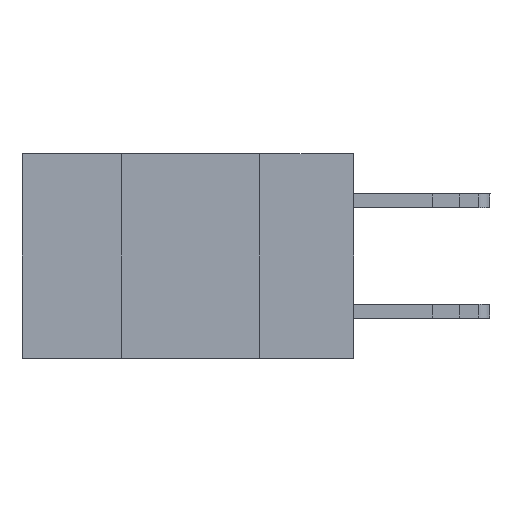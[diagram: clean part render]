
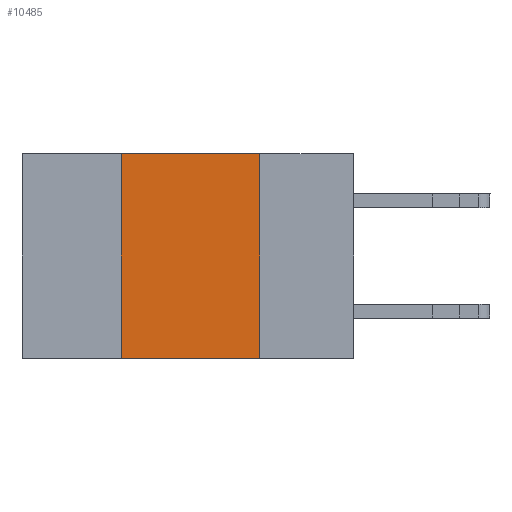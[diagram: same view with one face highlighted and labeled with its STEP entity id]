
A CAD part, left-side view. The second image highlights one B-rep face of the part: STEP entity #10485.
In plain terms, the highlighted planar face has unit normal (-1, 0, 0).
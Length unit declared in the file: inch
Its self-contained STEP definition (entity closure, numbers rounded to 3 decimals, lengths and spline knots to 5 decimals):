
#349 = CARTESIAN_POINT ( 'NONE',  ( 0., 0.17, 0. ) ) ;
#634 = CARTESIAN_POINT ( 'NONE',  ( 0., 0.17, 0. ) ) ;
#1159 = DIRECTION ( 'NONE',  ( 0., 0., 1. ) ) ;
#1369 = VECTOR ( 'NONE', #4876, 39.37008 ) ;
#2244 = CARTESIAN_POINT ( 'NONE',  ( 0., 0.42, -0.37 ) ) ;
#2671 = VERTEX_POINT ( 'NONE', #2244 ) ;
#2962 = EDGE_CURVE ( 'NONE', #2671, #11580, #12652, .T. ) ;
#3580 = DIRECTION ( 'NONE',  ( 1., 0., 0. ) ) ;
#3683 = AXIS2_PLACEMENT_3D ( 'NONE', #5428, #3580, #18559 ) ;
#3765 = DIRECTION ( 'NONE',  ( 0., 0., -1. ) ) ;
#4259 = EDGE_CURVE ( 'NONE', #2671, #16388, #11814, .T. ) ;
#4727 = ORIENTED_EDGE ( 'NONE', *, *, #13620, .F. ) ;
#4876 = DIRECTION ( 'NONE',  ( 0., -1., 0. ) ) ;
#5428 = CARTESIAN_POINT ( 'NONE',  ( 0., 0.6, 0. ) ) ;
#6842 = ORIENTED_EDGE ( 'NONE', *, *, #15157, .F. ) ;
#6956 = FACE_OUTER_BOUND ( 'NONE', #16777, .T. ) ;
#7000 = PLANE ( 'NONE',  #3683 ) ;
#7030 = VERTEX_POINT ( 'NONE', #634 ) ;
#10485 = ADVANCED_FACE ( 'NONE', ( #6956 ), #7000, .F. ) ;
#10540 = VECTOR ( 'NONE', #15843, 39.37008 ) ;
#11096 = CARTESIAN_POINT ( 'NONE',  ( 0., 0.6, -0.37 ) ) ;
#11365 = LINE ( 'NONE', #14636, #1369 ) ;
#11580 = VERTEX_POINT ( 'NONE', #15349 ) ;
#11814 = LINE ( 'NONE', #11096, #10540 ) ;
#12013 = ORIENTED_EDGE ( 'NONE', *, *, #2962, .F. ) ;
#12652 = LINE ( 'NONE', #19253, #17769 ) ;
#13620 = EDGE_CURVE ( 'NONE', #11580, #7030, #11365, .T. ) ;
#14636 = CARTESIAN_POINT ( 'NONE',  ( 0., 0.6, 0. ) ) ;
#15157 = EDGE_CURVE ( 'NONE', #7030, #16388, #16970, .T. ) ;
#15349 = CARTESIAN_POINT ( 'NONE',  ( 0., 0.42, 0. ) ) ;
#15436 = VECTOR ( 'NONE', #3765, 39.37008 ) ;
#15460 = ORIENTED_EDGE ( 'NONE', *, *, #4259, .T. ) ;
#15843 = DIRECTION ( 'NONE',  ( 0., -1., 0. ) ) ;
#16388 = VERTEX_POINT ( 'NONE', #17270 ) ;
#16777 = EDGE_LOOP ( 'NONE', ( #6842, #4727, #12013, #15460 ) ) ;
#16970 = LINE ( 'NONE', #349, #15436 ) ;
#17270 = CARTESIAN_POINT ( 'NONE',  ( 0., 0.17, -0.37 ) ) ;
#17769 = VECTOR ( 'NONE', #1159, 39.37008 ) ;
#18559 = DIRECTION ( 'NONE',  ( 0., 0., -1. ) ) ;
#19253 = CARTESIAN_POINT ( 'NONE',  ( 0., 0.42, 0. ) ) ;
